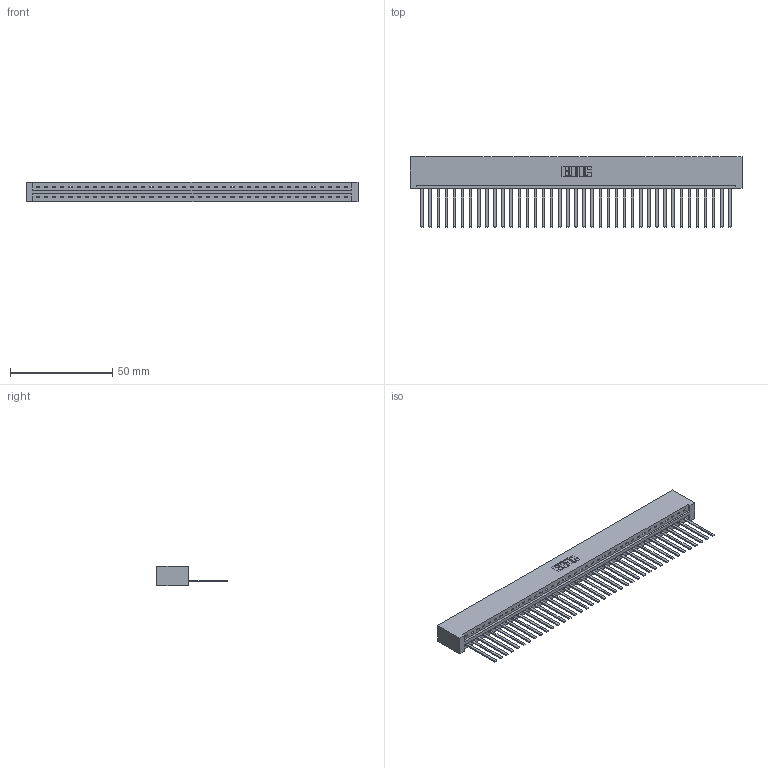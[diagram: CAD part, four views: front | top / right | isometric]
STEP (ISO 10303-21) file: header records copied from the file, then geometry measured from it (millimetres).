
FILE_DESCRIPTION (( 'STEP AP203' ), '1' );
FILE_NAME ('337-039-544-101.STEP', '2019-10-01T18:53:29', ( '' ), ( '' ), 'SwSTEP 2.0', 'SolidWorks 2016', '' );
FILE_SCHEMA (( 'CONFIG_CONTROL_DESIGN' ));
Length unit declared in the file: inch
Products named in the file (3): 337 Part_No Mounting Lugs; 337-039-544-101; 345-292-001_345-293-144
Assembly tree (40 placements, depth 2):
  337-039-544-101
    337 Part_No Mounting Lugs
    345-292-001_345-293-144  x39
Bounding box: 162.41 x 34.3 x 9.4 mm (x, y, z)
Volume: 18032.4 mm3; surface area: 20084.4 mm2
Topology: 40 solids, 40 shells, 2290 faces, 6917 edges, 4558 vertices
Faces by surface type: plane 1704, cylinder 586
Entity records: 28917 total; most frequent: CARTESIAN_POINT 5043, ORIENTED_EDGE 5018, DIRECTION 4239, EDGE_CURVE 2509, VECTOR 2393, LINE 2393, VERTEX_POINT 1670, AXIS2_PLACEMENT_3D 923
